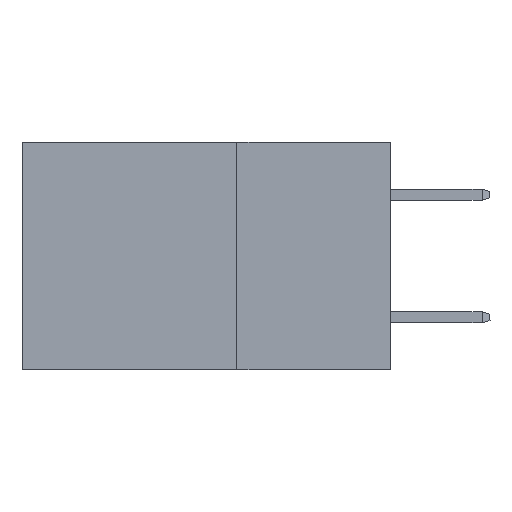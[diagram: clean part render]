
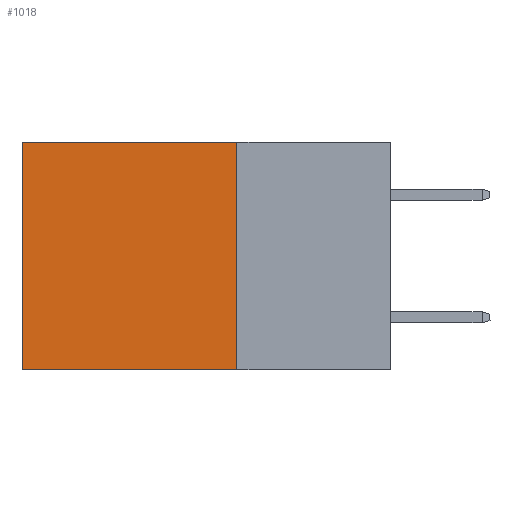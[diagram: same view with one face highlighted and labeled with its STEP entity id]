
A CAD part, left-side view. The second image highlights one B-rep face of the part: STEP entity #1018.
In plain terms, the highlighted planar face has unit normal (-1, 0, 0).
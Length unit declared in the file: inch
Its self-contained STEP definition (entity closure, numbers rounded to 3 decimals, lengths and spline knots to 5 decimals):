
#1018 = ADVANCED_FACE ( 'NONE', ( #12127 ), #7508, .F. ) ;
#1304 = DIRECTION ( 'NONE',  ( 0., 0., -1. ) ) ;
#1542 = AXIS2_PLACEMENT_3D ( 'NONE', #7535, #7872, #7080 ) ;
#1615 = CARTESIAN_POINT ( 'NONE',  ( 0.2875, 0.6, -0.37 ) ) ;
#2339 = EDGE_LOOP ( 'NONE', ( #7874, #5504, #18013, #4369 ) ) ;
#3846 = EDGE_CURVE ( 'NONE', #8968, #10649, #16981, .T. ) ;
#4369 = ORIENTED_EDGE ( 'NONE', *, *, #13478, .T. ) ;
#5138 = LINE ( 'NONE', #9744, #15100 ) ;
#5504 = ORIENTED_EDGE ( 'NONE', *, *, #13276, .F. ) ;
#6892 = DIRECTION ( 'NONE',  ( 0., 1., 0. ) ) ;
#6950 = CARTESIAN_POINT ( 'NONE',  ( 0.2875, 0.25, -0.37 ) ) ;
#7080 = DIRECTION ( 'NONE',  ( 0., 0., -1. ) ) ;
#7494 = VECTOR ( 'NONE', #6892, 39.37008 ) ;
#7508 = PLANE ( 'NONE',  #1542 ) ;
#7535 = CARTESIAN_POINT ( 'NONE',  ( 0.2875, 0.25, 0. ) ) ;
#7872 = DIRECTION ( 'NONE',  ( 1., 0., 0. ) ) ;
#7874 = ORIENTED_EDGE ( 'NONE', *, *, #3846, .T. ) ;
#7933 = LINE ( 'NONE', #6950, #7494 ) ;
#8417 = DIRECTION ( 'NONE',  ( 0., 0., -1. ) ) ;
#8754 = CARTESIAN_POINT ( 'NONE',  ( 0.2875, 0.25, 0. ) ) ;
#8968 = VERTEX_POINT ( 'NONE', #11310 ) ;
#9744 = CARTESIAN_POINT ( 'NONE',  ( 0.2875, 0.25, 0. ) ) ;
#10649 = VERTEX_POINT ( 'NONE', #1615 ) ;
#11310 = CARTESIAN_POINT ( 'NONE',  ( 0.2875, 0.6, 0. ) ) ;
#11348 = VECTOR ( 'NONE', #14112, 39.37008 ) ;
#11638 = VERTEX_POINT ( 'NONE', #16069 ) ;
#11967 = EDGE_CURVE ( 'NONE', #11638, #14768, #5138, .T. ) ;
#12127 = FACE_OUTER_BOUND ( 'NONE', #2339, .T. ) ;
#13276 = EDGE_CURVE ( 'NONE', #14768, #10649, #7933, .T. ) ;
#13465 = VECTOR ( 'NONE', #1304, 39.37008 ) ;
#13478 = EDGE_CURVE ( 'NONE', #11638, #8968, #15280, .T. ) ;
#14112 = DIRECTION ( 'NONE',  ( 0., 1., 0. ) ) ;
#14768 = VERTEX_POINT ( 'NONE', #17596 ) ;
#15100 = VECTOR ( 'NONE', #8417, 39.37008 ) ;
#15280 = LINE ( 'NONE', #8754, #11348 ) ;
#16069 = CARTESIAN_POINT ( 'NONE',  ( 0.2875, 0.25, 0. ) ) ;
#16523 = CARTESIAN_POINT ( 'NONE',  ( 0.2875, 0.6, 0. ) ) ;
#16981 = LINE ( 'NONE', #16523, #13465 ) ;
#17596 = CARTESIAN_POINT ( 'NONE',  ( 0.2875, 0.25, -0.37 ) ) ;
#18013 = ORIENTED_EDGE ( 'NONE', *, *, #11967, .F. ) ;
